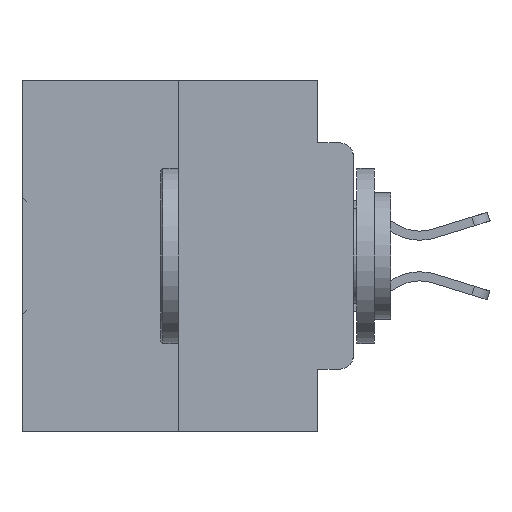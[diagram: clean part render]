
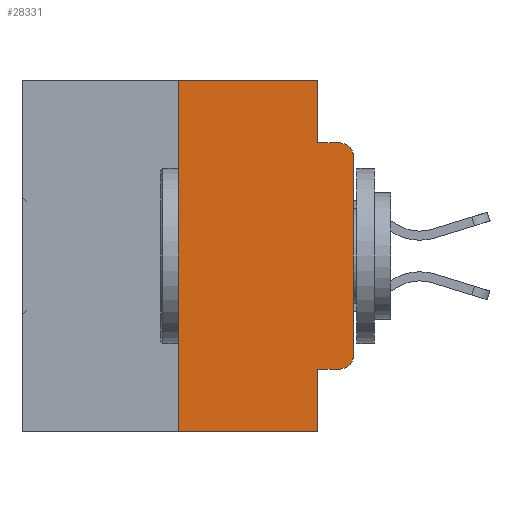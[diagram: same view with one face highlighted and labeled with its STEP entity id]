
A CAD part, left-side view. The second image highlights one B-rep face of the part: STEP entity #28331.
In plain terms, the highlighted planar face has unit normal (-1, 0, 0).
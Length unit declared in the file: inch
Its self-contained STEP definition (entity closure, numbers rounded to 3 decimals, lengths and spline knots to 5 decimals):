
#113 = EDGE_CURVE ( 'NONE', #14854, #33846, #11947, .T. ) ;
#304 = CARTESIAN_POINT ( 'NONE',  ( 0., 0.02, -0.3915 ) ) ;
#795 = ORIENTED_EDGE ( 'NONE', *, *, #2170, .F. ) ;
#832 = CARTESIAN_POINT ( 'NONE',  ( 0., 0.051, -0.4115 ) ) ;
#1328 = CARTESIAN_POINT ( 'NONE',  ( 0., 0.02, -0.1085 ) ) ;
#1410 = CARTESIAN_POINT ( 'NONE',  ( 0., 0.051, -0.4115 ) ) ;
#1820 = ORIENTED_EDGE ( 'NONE', *, *, #6727, .F. ) ;
#2170 = EDGE_CURVE ( 'NONE', #33846, #15920, #5104, .T. ) ;
#2631 = EDGE_CURVE ( 'NONE', #19278, #15446, #27493, .T. ) ;
#2721 = VECTOR ( 'NONE', #8803, 39.37008 ) ;
#2990 = DIRECTION ( 'NONE',  ( 0., 0., -1. ) ) ;
#3686 = CARTESIAN_POINT ( 'NONE',  ( 0., 0., 0. ) ) ;
#3963 = VECTOR ( 'NONE', #14186, 39.37008 ) ;
#4080 = DIRECTION ( 'NONE',  ( 0., -1., 0. ) ) ;
#4369 = CIRCLE ( 'NONE', #21838, 0.02 ) ;
#4454 = VECTOR ( 'NONE', #29685, 39.37008 ) ;
#4874 = CARTESIAN_POINT ( 'NONE',  ( 0., 0.051, -0.0885 ) ) ;
#5104 = LINE ( 'NONE', #20347, #25524 ) ;
#5860 = VERTEX_POINT ( 'NONE', #13267 ) ;
#5953 = EDGE_CURVE ( 'NONE', #20416, #19942, #4369, .T. ) ;
#6127 = CARTESIAN_POINT ( 'NONE',  ( 0., 0.051, -0.0885 ) ) ;
#6727 = EDGE_CURVE ( 'NONE', #31969, #15446, #10667, .T. ) ;
#6930 = VECTOR ( 'NONE', #4080, 39.37008 ) ;
#7076 = AXIS2_PLACEMENT_3D ( 'NONE', #1328, #24255, #24146 ) ;
#7733 = CARTESIAN_POINT ( 'NONE',  ( 0., 0., -0.1085 ) ) ;
#8651 = CARTESIAN_POINT ( 'NONE',  ( 0., 0.02, -0.0885 ) ) ;
#8803 = DIRECTION ( 'NONE',  ( 0., -1., 0. ) ) ;
#9187 = CARTESIAN_POINT ( 'NONE',  ( 0., 0.25, 0. ) ) ;
#9205 = DIRECTION ( 'NONE',  ( 0., 0., 1. ) ) ;
#10333 = CARTESIAN_POINT ( 'NONE',  ( 0., 0., -0.3915 ) ) ;
#10571 = PLANE ( 'NONE',  #25735 ) ;
#10667 = LINE ( 'NONE', #6127, #2721 ) ;
#11405 = EDGE_CURVE ( 'NONE', #20188, #5860, #26641, .T. ) ;
#11947 = LINE ( 'NONE', #9187, #3963 ) ;
#13267 = CARTESIAN_POINT ( 'NONE',  ( 0., 0.051, -0.5 ) ) ;
#13975 = CARTESIAN_POINT ( 'NONE',  ( 0., 0.25, 0. ) ) ;
#14186 = DIRECTION ( 'NONE',  ( 0., 0., 1. ) ) ;
#14337 = VECTOR ( 'NONE', #9205, 39.37008 ) ;
#14854 = VERTEX_POINT ( 'NONE', #16817 ) ;
#15006 = ORIENTED_EDGE ( 'NONE', *, *, #113, .F. ) ;
#15035 = ORIENTED_EDGE ( 'NONE', *, *, #5953, .T. ) ;
#15446 = VERTEX_POINT ( 'NONE', #8651 ) ;
#15920 = VERTEX_POINT ( 'NONE', #28464 ) ;
#15922 = DIRECTION ( 'NONE',  ( 1., 0., 0. ) ) ;
#16817 = CARTESIAN_POINT ( 'NONE',  ( 0., 0.25, -0.5 ) ) ;
#17750 = CARTESIAN_POINT ( 'NONE',  ( 0., 0.02, -0.4115 ) ) ;
#18501 = CARTESIAN_POINT ( 'NONE',  ( 0., 0.473, 0. ) ) ;
#18674 = LINE ( 'NONE', #27067, #4454 ) ;
#18789 = VECTOR ( 'NONE', #23831, 39.37008 ) ;
#18979 = DIRECTION ( 'NONE',  ( -1., 0., 0. ) ) ;
#19278 = VERTEX_POINT ( 'NONE', #7733 ) ;
#19321 = EDGE_LOOP ( 'NONE', ( #20601, #29237, #1820, #24980, #795, #15006, #27858, #22514, #25015, #15035 ) ) ;
#19942 = VERTEX_POINT ( 'NONE', #10333 ) ;
#20097 = DIRECTION ( 'NONE',  ( 0., -1., 0. ) ) ;
#20188 = VERTEX_POINT ( 'NONE', #832 ) ;
#20314 = EDGE_CURVE ( 'NONE', #20188, #20416, #28072, .T. ) ;
#20347 = CARTESIAN_POINT ( 'NONE',  ( 0., 0.473, 0. ) ) ;
#20416 = VERTEX_POINT ( 'NONE', #17750 ) ;
#20601 = ORIENTED_EDGE ( 'NONE', *, *, #27987, .T. ) ;
#21166 = CARTESIAN_POINT ( 'NONE',  ( 0., 0.051, 0. ) ) ;
#21409 = LINE ( 'NONE', #3686, #14337 ) ;
#21838 = AXIS2_PLACEMENT_3D ( 'NONE', #304, #18979, #2990 ) ;
#22455 = EDGE_CURVE ( 'NONE', #14854, #5860, #34051, .T. ) ;
#22514 = ORIENTED_EDGE ( 'NONE', *, *, #11405, .F. ) ;
#23831 = DIRECTION ( 'NONE',  ( 0., 0., -1. ) ) ;
#23875 = FACE_OUTER_BOUND ( 'NONE', #19321, .T. ) ;
#24146 = DIRECTION ( 'NONE',  ( 0., 0., -1. ) ) ;
#24255 = DIRECTION ( 'NONE',  ( -1., 0., 0. ) ) ;
#24980 = ORIENTED_EDGE ( 'NONE', *, *, #32184, .F. ) ;
#25015 = ORIENTED_EDGE ( 'NONE', *, *, #20314, .T. ) ;
#25524 = VECTOR ( 'NONE', #20097, 39.37008 ) ;
#25549 = VECTOR ( 'NONE', #31466, 39.37008 ) ;
#25735 = AXIS2_PLACEMENT_3D ( 'NONE', #18501, #15922, #34290 ) ;
#26641 = LINE ( 'NONE', #21166, #18789 ) ;
#27067 = CARTESIAN_POINT ( 'NONE',  ( 0., 0.051, 0. ) ) ;
#27493 = CIRCLE ( 'NONE', #7076, 0.02 ) ;
#27858 = ORIENTED_EDGE ( 'NONE', *, *, #22455, .T. ) ;
#27987 = EDGE_CURVE ( 'NONE', #19942, #19278, #21409, .T. ) ;
#28072 = LINE ( 'NONE', #1410, #6930 ) ;
#28331 = ADVANCED_FACE ( 'NONE', ( #23875 ), #10571, .F. ) ;
#28464 = CARTESIAN_POINT ( 'NONE',  ( 0., 0.051, 0. ) ) ;
#29237 = ORIENTED_EDGE ( 'NONE', *, *, #2631, .T. ) ;
#29685 = DIRECTION ( 'NONE',  ( 0., 0., -1. ) ) ;
#31466 = DIRECTION ( 'NONE',  ( 0., -1., 0. ) ) ;
#31578 = CARTESIAN_POINT ( 'NONE',  ( 0., 0.473, -0.5 ) ) ;
#31969 = VERTEX_POINT ( 'NONE', #4874 ) ;
#32184 = EDGE_CURVE ( 'NONE', #15920, #31969, #18674, .T. ) ;
#33846 = VERTEX_POINT ( 'NONE', #13975 ) ;
#34051 = LINE ( 'NONE', #31578, #25549 ) ;
#34290 = DIRECTION ( 'NONE',  ( 0., 0., -1. ) ) ;
